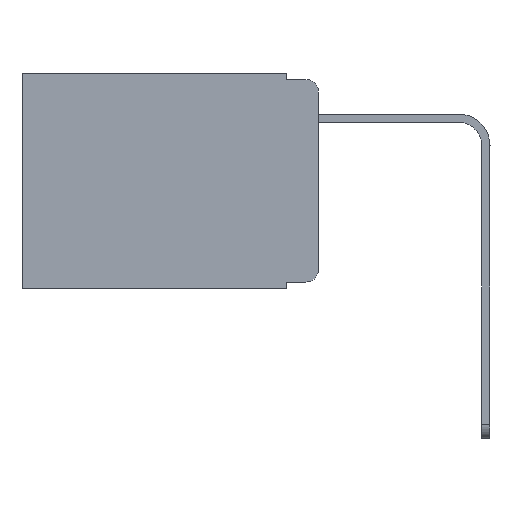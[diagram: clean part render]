
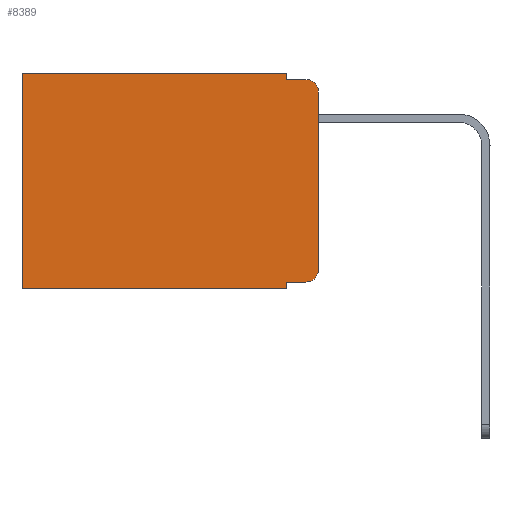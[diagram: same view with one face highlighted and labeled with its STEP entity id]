
A CAD part, left-side view. The second image highlights one B-rep face of the part: STEP entity #8389.
In plain terms, the highlighted planar face has unit normal (-1, 0, 0).
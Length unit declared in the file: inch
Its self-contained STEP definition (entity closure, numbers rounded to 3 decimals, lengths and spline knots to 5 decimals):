
#172 = CARTESIAN_POINT ( 'NONE',  ( 0.298, 0.051, -0.343 ) ) ;
#202 = LINE ( 'NONE', #3314, #8322 ) ;
#443 = EDGE_CURVE ( 'NONE', #4671, #8411, #202, .T. ) ;
#466 = DIRECTION ( 'NONE',  ( 0., 0., -1. ) ) ;
#488 = DIRECTION ( 'NONE',  ( -1., 0., 0. ) ) ;
#723 = LINE ( 'NONE', #3365, #3153 ) ;
#789 = CARTESIAN_POINT ( 'NONE',  ( 0.298, 0., 0. ) ) ;
#835 = DIRECTION ( 'NONE',  ( 0., 1., 0. ) ) ;
#953 = DIRECTION ( 'NONE',  ( 0., -1., 0. ) ) ;
#961 = ORIENTED_EDGE ( 'NONE', *, *, #1987, .T. ) ;
#1102 = ORIENTED_EDGE ( 'NONE', *, *, #4782, .F. ) ;
#1461 = EDGE_CURVE ( 'NONE', #2681, #9472, #6927, .T. ) ;
#1492 = DIRECTION ( 'NONE',  ( 0., -1., 0. ) ) ;
#1517 = EDGE_CURVE ( 'NONE', #4671, #4628, #3784, .T. ) ;
#1592 = ORIENTED_EDGE ( 'NONE', *, *, #1517, .T. ) ;
#1648 = DIRECTION ( 'NONE',  ( 0., 0., -1. ) ) ;
#1987 = EDGE_CURVE ( 'NONE', #2681, #2051, #723, .T. ) ;
#2051 = VERTEX_POINT ( 'NONE', #8814 ) ;
#2529 = DIRECTION ( 'NONE',  ( -1., 0., 0. ) ) ;
#2558 = CARTESIAN_POINT ( 'NONE',  ( 0.298, 0.02, -0.03 ) ) ;
#2681 = VERTEX_POINT ( 'NONE', #3796 ) ;
#2764 = ORIENTED_EDGE ( 'NONE', *, *, #8203, .F. ) ;
#2808 = VERTEX_POINT ( 'NONE', #3984 ) ;
#2812 = CARTESIAN_POINT ( 'NONE',  ( 0.298, 0.473, 0. ) ) ;
#2852 = CARTESIAN_POINT ( 'NONE',  ( 0.298, 0., -0.03 ) ) ;
#3153 = VECTOR ( 'NONE', #953, 39.37008 ) ;
#3260 = VECTOR ( 'NONE', #1492, 39.37008 ) ;
#3277 = PLANE ( 'NONE',  #3732 ) ;
#3314 = CARTESIAN_POINT ( 'NONE',  ( 0.298, 0.051, 0. ) ) ;
#3365 = CARTESIAN_POINT ( 'NONE',  ( 0.298, 0.051, -0.333 ) ) ;
#3689 = CARTESIAN_POINT ( 'NONE',  ( 0.298, 0.051, 0. ) ) ;
#3732 = AXIS2_PLACEMENT_3D ( 'NONE', #6354, #8788, #4055 ) ;
#3784 = LINE ( 'NONE', #789, #4391 ) ;
#3796 = CARTESIAN_POINT ( 'NONE',  ( 0.298, 0.051, -0.333 ) ) ;
#3940 = VERTEX_POINT ( 'NONE', #6145 ) ;
#3984 = CARTESIAN_POINT ( 'NONE',  ( 0.298, 0., -0.313 ) ) ;
#4008 = CARTESIAN_POINT ( 'NONE',  ( 0.298, 0.051, 0. ) ) ;
#4055 = DIRECTION ( 'NONE',  ( 0., 0., -1. ) ) ;
#4182 = LINE ( 'NONE', #10151, #5181 ) ;
#4317 = FACE_OUTER_BOUND ( 'NONE', #9629, .T. ) ;
#4391 = VECTOR ( 'NONE', #7269, 39.37008 ) ;
#4483 = AXIS2_PLACEMENT_3D ( 'NONE', #2558, #2529, #1648 ) ;
#4628 = VERTEX_POINT ( 'NONE', #4738 ) ;
#4671 = VERTEX_POINT ( 'NONE', #4008 ) ;
#4738 = CARTESIAN_POINT ( 'NONE',  ( 0.298, 0.473, 0. ) ) ;
#4767 = VERTEX_POINT ( 'NONE', #2852 ) ;
#4782 = EDGE_CURVE ( 'NONE', #4767, #2808, #6178, .T. ) ;
#4988 = EDGE_CURVE ( 'NONE', #4767, #3940, #7714, .T. ) ;
#5013 = ORIENTED_EDGE ( 'NONE', *, *, #1461, .F. ) ;
#5101 = DIRECTION ( 'NONE',  ( 0., 0., -1. ) ) ;
#5147 = CARTESIAN_POINT ( 'NONE',  ( 0.298, 0., 0. ) ) ;
#5181 = VECTOR ( 'NONE', #835, 39.37008 ) ;
#5315 = AXIS2_PLACEMENT_3D ( 'NONE', #9955, #488, #5101 ) ;
#5378 = CARTESIAN_POINT ( 'NONE',  ( 0.298, 0.051, -0.01 ) ) ;
#5411 = DIRECTION ( 'NONE',  ( 0., 0., -1. ) ) ;
#5693 = CARTESIAN_POINT ( 'NONE',  ( 0.298, 0.051, -0.01 ) ) ;
#5844 = VERTEX_POINT ( 'NONE', #6112 ) ;
#5920 = VECTOR ( 'NONE', #466, 39.37008 ) ;
#5937 = VECTOR ( 'NONE', #5411, 39.37008 ) ;
#6112 = CARTESIAN_POINT ( 'NONE',  ( 0.298, 0.473, -0.343 ) ) ;
#6145 = CARTESIAN_POINT ( 'NONE',  ( 0.298, 0.02, -0.01 ) ) ;
#6178 = LINE ( 'NONE', #5147, #5920 ) ;
#6354 = CARTESIAN_POINT ( 'NONE',  ( 0.298, 0., 0. ) ) ;
#6537 = LINE ( 'NONE', #2812, #7054 ) ;
#6705 = ORIENTED_EDGE ( 'NONE', *, *, #443, .F. ) ;
#6857 = ORIENTED_EDGE ( 'NONE', *, *, #7654, .F. ) ;
#6927 = LINE ( 'NONE', #3689, #5937 ) ;
#6965 = EDGE_CURVE ( 'NONE', #4628, #5844, #6537, .T. ) ;
#7054 = VECTOR ( 'NONE', #7467, 39.37008 ) ;
#7067 = ORIENTED_EDGE ( 'NONE', *, *, #8616, .T. ) ;
#7269 = DIRECTION ( 'NONE',  ( 0., 1., 0. ) ) ;
#7467 = DIRECTION ( 'NONE',  ( 0., 0., -1. ) ) ;
#7654 = EDGE_CURVE ( 'NONE', #8411, #3940, #9186, .T. ) ;
#7714 = CIRCLE ( 'NONE', #4483, 0.02 ) ;
#7755 = ORIENTED_EDGE ( 'NONE', *, *, #6965, .T. ) ;
#8203 = EDGE_CURVE ( 'NONE', #9472, #5844, #4182, .T. ) ;
#8322 = VECTOR ( 'NONE', #9445, 39.37008 ) ;
#8389 = ADVANCED_FACE ( 'NONE', ( #4317 ), #3277, .F. ) ;
#8411 = VERTEX_POINT ( 'NONE', #5693 ) ;
#8616 = EDGE_CURVE ( 'NONE', #2051, #2808, #9362, .T. ) ;
#8788 = DIRECTION ( 'NONE',  ( 1., 0., 0. ) ) ;
#8814 = CARTESIAN_POINT ( 'NONE',  ( 0.298, 0.02, -0.333 ) ) ;
#9186 = LINE ( 'NONE', #5378, #3260 ) ;
#9362 = CIRCLE ( 'NONE', #5315, 0.02 ) ;
#9445 = DIRECTION ( 'NONE',  ( 0., 0., -1. ) ) ;
#9472 = VERTEX_POINT ( 'NONE', #172 ) ;
#9572 = ORIENTED_EDGE ( 'NONE', *, *, #4988, .T. ) ;
#9629 = EDGE_LOOP ( 'NONE', ( #1102, #9572, #6857, #6705, #1592, #7755, #2764, #5013, #961, #7067 ) ) ;
#9955 = CARTESIAN_POINT ( 'NONE',  ( 0.298, 0.02, -0.313 ) ) ;
#10151 = CARTESIAN_POINT ( 'NONE',  ( 0.298, 0., -0.343 ) ) ;
